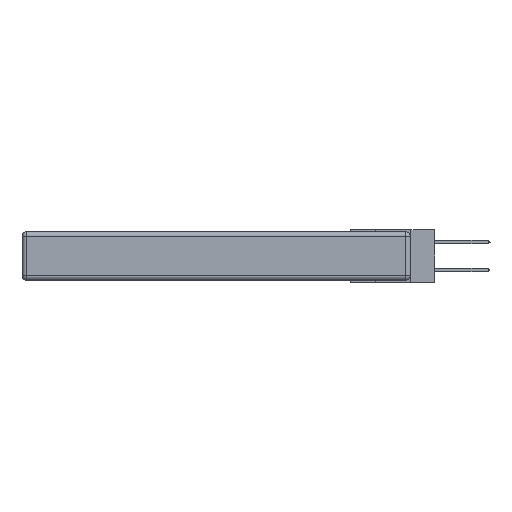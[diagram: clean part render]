
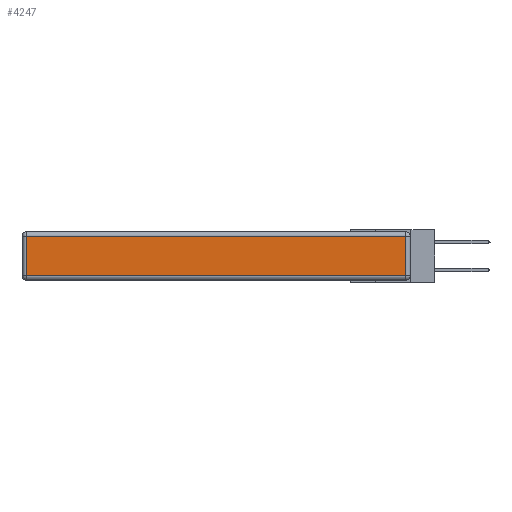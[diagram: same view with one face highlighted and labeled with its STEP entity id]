
A CAD part, left-side view. The second image highlights one B-rep face of the part: STEP entity #4247.
In plain terms, the highlighted planar face has unit normal (-1, 0, 0).
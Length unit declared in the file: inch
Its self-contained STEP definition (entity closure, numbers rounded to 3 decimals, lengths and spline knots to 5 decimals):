
#50 = VERTEX_POINT ( 'NONE', #10108 ) ;
#262 = CARTESIAN_POINT ( 'NONE',  ( 0., 2.72, -0.343 ) ) ;
#686 = CARTESIAN_POINT ( 'NONE',  ( 0., 0.03, -0.03 ) ) ;
#726 = EDGE_CURVE ( 'NONE', #11833, #10909, #14069, .T. ) ;
#1459 = EDGE_CURVE ( 'NONE', #1583, #11833, #20234, .T. ) ;
#1583 = VERTEX_POINT ( 'NONE', #3073 ) ;
#3073 = CARTESIAN_POINT ( 'NONE',  ( 0., 2.72, -0.313 ) ) ;
#3374 = LINE ( 'NONE', #262, #22919 ) ;
#4247 = ADVANCED_FACE ( 'NONE', ( #16882 ), #10685, .T. ) ;
#4341 = ORIENTED_EDGE ( 'NONE', *, *, #14184, .T. ) ;
#5166 = LINE ( 'NONE', #19114, #19672 ) ;
#5595 = EDGE_LOOP ( 'NONE', ( #22816, #22923, #21282, #4341 ) ) ;
#5855 = DIRECTION ( 'NONE',  ( 0., 1., 0. ) ) ;
#7024 = CARTESIAN_POINT ( 'NONE',  ( 0., 0.03, -0.313 ) ) ;
#9912 = DIRECTION ( 'NONE',  ( 0., 0., -1. ) ) ;
#10108 = CARTESIAN_POINT ( 'NONE',  ( 0., 2.72, -0.03 ) ) ;
#10392 = CARTESIAN_POINT ( 'NONE',  ( 0., 0., -0.313 ) ) ;
#10685 = PLANE ( 'NONE',  #22693 ) ;
#10909 = VERTEX_POINT ( 'NONE', #686 ) ;
#11833 = VERTEX_POINT ( 'NONE', #7024 ) ;
#14069 = LINE ( 'NONE', #15264, #18507 ) ;
#14184 = EDGE_CURVE ( 'NONE', #50, #1583, #3374, .T. ) ;
#14504 = CARTESIAN_POINT ( 'NONE',  ( 0., 0., -0.343 ) ) ;
#15264 = CARTESIAN_POINT ( 'NONE',  ( 0., 0.03, -0.343 ) ) ;
#16159 = DIRECTION ( 'NONE',  ( 0., 0., 1. ) ) ;
#16882 = FACE_OUTER_BOUND ( 'NONE', #5595, .T. ) ;
#18327 = DIRECTION ( 'NONE',  ( -1., 0., 0. ) ) ;
#18507 = VECTOR ( 'NONE', #20648, 39.37008 ) ;
#18685 = EDGE_CURVE ( 'NONE', #10909, #50, #5166, .T. ) ;
#19114 = CARTESIAN_POINT ( 'NONE',  ( 0., 2.75, -0.03 ) ) ;
#19633 = VECTOR ( 'NONE', #23413, 39.37008 ) ;
#19672 = VECTOR ( 'NONE', #5855, 39.37008 ) ;
#20234 = LINE ( 'NONE', #10392, #19633 ) ;
#20648 = DIRECTION ( 'NONE',  ( 0., 0., 1. ) ) ;
#21282 = ORIENTED_EDGE ( 'NONE', *, *, #18685, .T. ) ;
#22693 = AXIS2_PLACEMENT_3D ( 'NONE', #14504, #18327, #16159 ) ;
#22816 = ORIENTED_EDGE ( 'NONE', *, *, #1459, .T. ) ;
#22919 = VECTOR ( 'NONE', #9912, 39.37008 ) ;
#22923 = ORIENTED_EDGE ( 'NONE', *, *, #726, .T. ) ;
#23413 = DIRECTION ( 'NONE',  ( 0., -1., 0. ) ) ;
